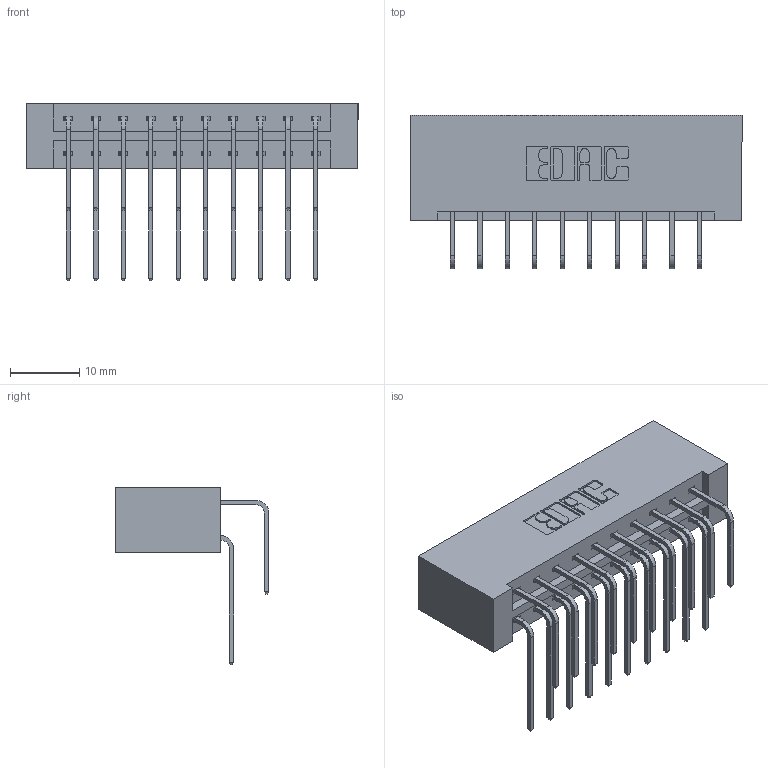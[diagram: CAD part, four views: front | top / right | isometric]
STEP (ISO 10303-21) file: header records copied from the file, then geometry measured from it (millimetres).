
FILE_DESCRIPTION (( 'STEP AP203' ), '1' );
FILE_NAME ('333-020-558-201.STEP', '2018-08-02T00:31:49', ( '' ), ( '' ), 'SwSTEP 2.0', 'SolidWorks 2016', '' );
FILE_SCHEMA (( 'CONFIG_CONTROL_DESIGN' ));
Length unit declared in the file: inch
Products named in the file (4): 333-020-558-201; 333 Part_Lugless; 345-292-001_558 559 Tail - 1; 345-292-001_558 Tail - 2
Assembly tree (21 placements, depth 2):
  333-020-558-201
    333 Part_Lugless
    345-292-001_558 559 Tail - 1  x10
    345-292-001_558 Tail - 2  x10
Bounding box: 47.88 x 22.17 x 25.53 mm (x, y, z)
Volume: 5336.5 mm3; surface area: 6564.3 mm2
Topology: 21 solids, 21 shells, 1186 faces, 3507 edges, 2310 vertices
Faces by surface type: plane 826, cylinder 360
Entity records: 12079 total; most frequent: CARTESIAN_POINT 2089, ORIENTED_EDGE 1974, DIRECTION 1815, EDGE_CURVE 987, LINE 827, VECTOR 827, VERTEX_POINT 654, AXIS2_PLACEMENT_3D 494
